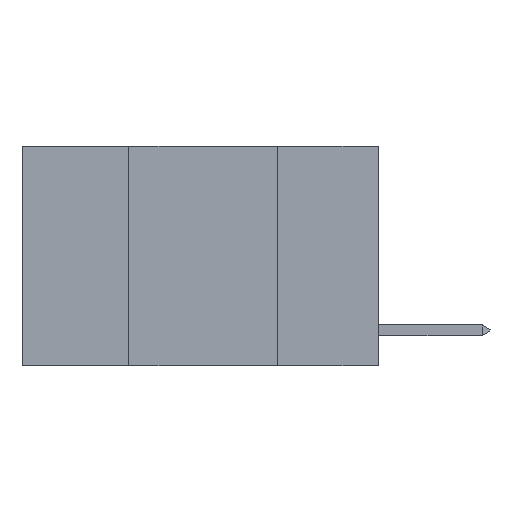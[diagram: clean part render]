
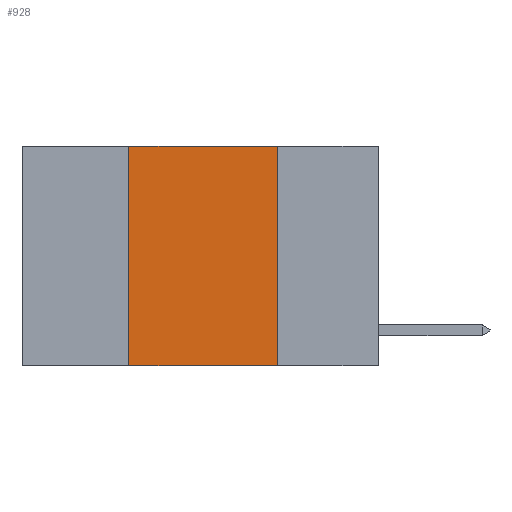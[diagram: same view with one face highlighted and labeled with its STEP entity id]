
A CAD part, left-side view. The second image highlights one B-rep face of the part: STEP entity #928.
In plain terms, the highlighted planar face has unit normal (-1, 0, 0).
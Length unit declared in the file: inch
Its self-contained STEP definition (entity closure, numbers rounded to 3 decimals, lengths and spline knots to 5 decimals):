
#259 = LINE ( 'NONE', #15019, #9878 ) ;
#928 = ADVANCED_FACE ( 'NONE', ( #18107 ), #19699, .F. ) ;
#1891 = VECTOR ( 'NONE', #10950, 39.37008 ) ;
#2775 = CARTESIAN_POINT ( 'NONE',  ( 0., 0.6, 0. ) ) ;
#2959 = CARTESIAN_POINT ( 'NONE',  ( 0., 0.42, 0. ) ) ;
#3040 = VECTOR ( 'NONE', #19212, 39.37008 ) ;
#3826 = ORIENTED_EDGE ( 'NONE', *, *, #10915, .T. ) ;
#4647 = ORIENTED_EDGE ( 'NONE', *, *, #20616, .F. ) ;
#6047 = EDGE_CURVE ( 'NONE', #11043, #17849, #6123, .T. ) ;
#6123 = LINE ( 'NONE', #19094, #3040 ) ;
#6560 = LINE ( 'NONE', #2775, #20385 ) ;
#6627 = CARTESIAN_POINT ( 'NONE',  ( 0., 0.17, -0.37 ) ) ;
#9411 = DIRECTION ( 'NONE',  ( 0., 0., -1. ) ) ;
#9878 = VECTOR ( 'NONE', #9411, 39.37008 ) ;
#10915 = EDGE_CURVE ( 'NONE', #11043, #19125, #22056, .T. ) ;
#10950 = DIRECTION ( 'NONE',  ( 0., -1., 0. ) ) ;
#11043 = VERTEX_POINT ( 'NONE', #18658 ) ;
#11499 = VERTEX_POINT ( 'NONE', #16255 ) ;
#11688 = ORIENTED_EDGE ( 'NONE', *, *, #6047, .F. ) ;
#12320 = EDGE_LOOP ( 'NONE', ( #17256, #4647, #11688, #3826 ) ) ;
#13131 = CARTESIAN_POINT ( 'NONE',  ( 0., 0.6, -0.37 ) ) ;
#13740 = DIRECTION ( 'NONE',  ( 0., -1., 0. ) ) ;
#15019 = CARTESIAN_POINT ( 'NONE',  ( 0., 0.17, 0. ) ) ;
#16255 = CARTESIAN_POINT ( 'NONE',  ( 0., 0.17, 0. ) ) ;
#17256 = ORIENTED_EDGE ( 'NONE', *, *, #23433, .F. ) ;
#17526 = AXIS2_PLACEMENT_3D ( 'NONE', #18225, #21505, #23826 ) ;
#17849 = VERTEX_POINT ( 'NONE', #2959 ) ;
#18107 = FACE_OUTER_BOUND ( 'NONE', #12320, .T. ) ;
#18225 = CARTESIAN_POINT ( 'NONE',  ( 0., 0.6, 0. ) ) ;
#18658 = CARTESIAN_POINT ( 'NONE',  ( 0., 0.42, -0.37 ) ) ;
#19094 = CARTESIAN_POINT ( 'NONE',  ( 0., 0.42, 0. ) ) ;
#19125 = VERTEX_POINT ( 'NONE', #6627 ) ;
#19212 = DIRECTION ( 'NONE',  ( 0., 0., 1. ) ) ;
#19699 = PLANE ( 'NONE',  #17526 ) ;
#20385 = VECTOR ( 'NONE', #13740, 39.37008 ) ;
#20616 = EDGE_CURVE ( 'NONE', #17849, #11499, #6560, .T. ) ;
#21505 = DIRECTION ( 'NONE',  ( 1., 0., 0. ) ) ;
#22056 = LINE ( 'NONE', #13131, #1891 ) ;
#23433 = EDGE_CURVE ( 'NONE', #11499, #19125, #259, .T. ) ;
#23826 = DIRECTION ( 'NONE',  ( 0., 0., -1. ) ) ;
